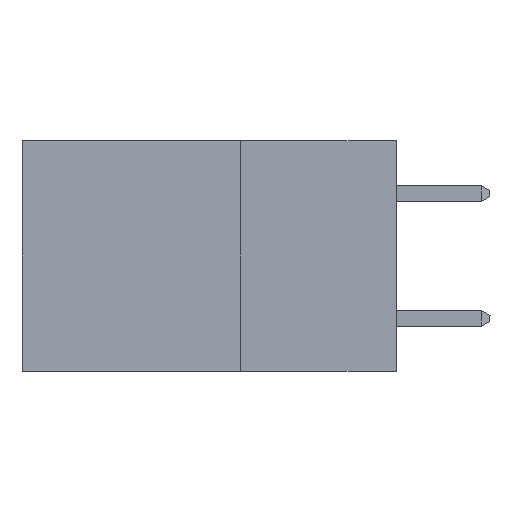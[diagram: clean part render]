
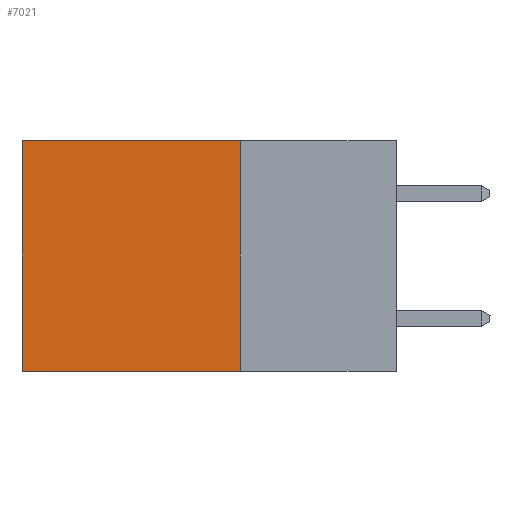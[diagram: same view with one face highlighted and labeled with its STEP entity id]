
A CAD part, left-side view. The second image highlights one B-rep face of the part: STEP entity #7021.
In plain terms, the highlighted planar face has unit normal (-1, 0, 0).
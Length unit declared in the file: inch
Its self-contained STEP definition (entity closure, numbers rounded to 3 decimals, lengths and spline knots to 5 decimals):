
#369 = LINE ( 'NONE', #7918, #7357 ) ;
#496 = PLANE ( 'NONE',  #3435 ) ;
#620 = LINE ( 'NONE', #679, #1698 ) ;
#639 = CARTESIAN_POINT ( 'NONE',  ( 0.298, 0.25, -0.37 ) ) ;
#679 = CARTESIAN_POINT ( 'NONE',  ( 0.298, 0.25, 0. ) ) ;
#953 = VERTEX_POINT ( 'NONE', #3412 ) ;
#1007 = CARTESIAN_POINT ( 'NONE',  ( 0.298, 0.6, 0. ) ) ;
#1572 = DIRECTION ( 'NONE',  ( 0., 0., -1. ) ) ;
#1698 = VECTOR ( 'NONE', #1572, 39.37008 ) ;
#1925 = EDGE_CURVE ( 'NONE', #6388, #10418, #4163, .T. ) ;
#2357 = DIRECTION ( 'NONE',  ( 0., 1., 0. ) ) ;
#2497 = EDGE_LOOP ( 'NONE', ( #3893, #3197, #4286, #10686 ) ) ;
#3121 = DIRECTION ( 'NONE',  ( 0., 0., -1. ) ) ;
#3197 = ORIENTED_EDGE ( 'NONE', *, *, #8762, .F. ) ;
#3412 = CARTESIAN_POINT ( 'NONE',  ( 0.298, 0.25, -0.37 ) ) ;
#3435 = AXIS2_PLACEMENT_3D ( 'NONE', #6547, #3936, #3121 ) ;
#3634 = DIRECTION ( 'NONE',  ( 0., 1., 0. ) ) ;
#3893 = ORIENTED_EDGE ( 'NONE', *, *, #1925, .T. ) ;
#3936 = DIRECTION ( 'NONE',  ( 1., 0., 0. ) ) ;
#4163 = LINE ( 'NONE', #1007, #9725 ) ;
#4286 = ORIENTED_EDGE ( 'NONE', *, *, #7157, .F. ) ;
#5108 = LINE ( 'NONE', #639, #10459 ) ;
#5767 = EDGE_CURVE ( 'NONE', #10709, #6388, #369, .T. ) ;
#6388 = VERTEX_POINT ( 'NONE', #8347 ) ;
#6547 = CARTESIAN_POINT ( 'NONE',  ( 0.298, 0.25, 0. ) ) ;
#7021 = ADVANCED_FACE ( 'NONE', ( #9383 ), #496, .F. ) ;
#7157 = EDGE_CURVE ( 'NONE', #10709, #953, #620, .T. ) ;
#7357 = VECTOR ( 'NONE', #3634, 39.37008 ) ;
#7799 = DIRECTION ( 'NONE',  ( 0., 0., -1. ) ) ;
#7918 = CARTESIAN_POINT ( 'NONE',  ( 0.298, 0.25, 0. ) ) ;
#8347 = CARTESIAN_POINT ( 'NONE',  ( 0.298, 0.6, 0. ) ) ;
#8762 = EDGE_CURVE ( 'NONE', #953, #10418, #5108, .T. ) ;
#9383 = FACE_OUTER_BOUND ( 'NONE', #2497, .T. ) ;
#9725 = VECTOR ( 'NONE', #7799, 39.37008 ) ;
#9767 = CARTESIAN_POINT ( 'NONE',  ( 0.298, 0.25, 0. ) ) ;
#10418 = VERTEX_POINT ( 'NONE', #10899 ) ;
#10459 = VECTOR ( 'NONE', #2357, 39.37008 ) ;
#10686 = ORIENTED_EDGE ( 'NONE', *, *, #5767, .T. ) ;
#10709 = VERTEX_POINT ( 'NONE', #9767 ) ;
#10899 = CARTESIAN_POINT ( 'NONE',  ( 0.298, 0.6, -0.37 ) ) ;
